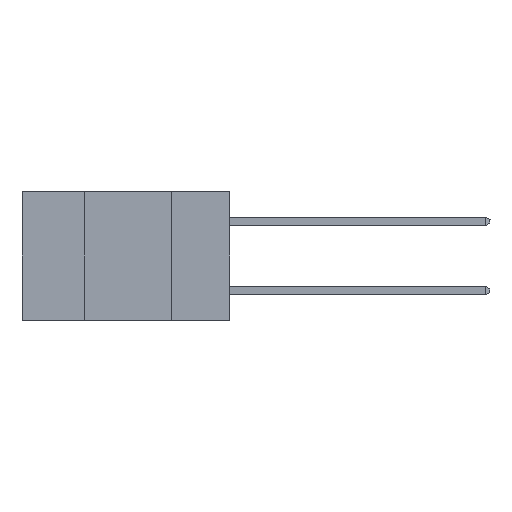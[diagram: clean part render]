
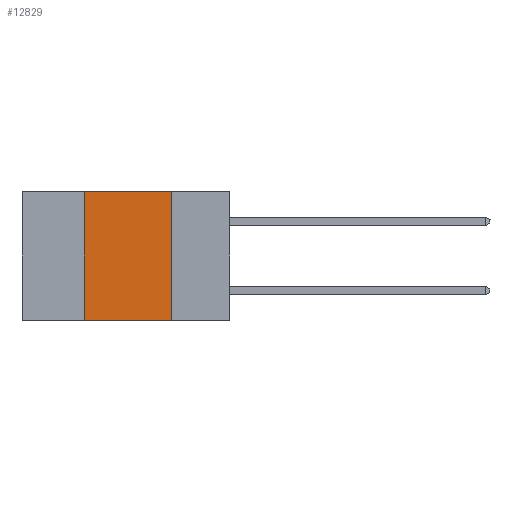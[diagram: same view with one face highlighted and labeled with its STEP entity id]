
A CAD part, left-side view. The second image highlights one B-rep face of the part: STEP entity #12829.
In plain terms, the highlighted planar face has unit normal (-1, 0, 0).
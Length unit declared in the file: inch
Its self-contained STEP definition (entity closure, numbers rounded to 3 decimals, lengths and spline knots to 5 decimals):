
#704 = DIRECTION ( 'NONE',  ( 0., 0., 1. ) ) ;
#852 = EDGE_CURVE ( 'NONE', #13391, #5458, #10496, .T. ) ;
#1098 = FACE_OUTER_BOUND ( 'NONE', #7113, .T. ) ;
#1735 = CARTESIAN_POINT ( 'NONE',  ( 0., 0.17, -0.37 ) ) ;
#2608 = ORIENTED_EDGE ( 'NONE', *, *, #852, .F. ) ;
#2869 = VERTEX_POINT ( 'NONE', #13666 ) ;
#3150 = VECTOR ( 'NONE', #5096, 39.37008 ) ;
#3332 = VERTEX_POINT ( 'NONE', #1735 ) ;
#4111 = CARTESIAN_POINT ( 'NONE',  ( 0., 0.6, 0. ) ) ;
#4150 = LINE ( 'NONE', #6909, #11896 ) ;
#4153 = DIRECTION ( 'NONE',  ( 1., 0., 0. ) ) ;
#5096 = DIRECTION ( 'NONE',  ( 0., -1., 0. ) ) ;
#5458 = VERTEX_POINT ( 'NONE', #6648 ) ;
#5935 = ORIENTED_EDGE ( 'NONE', *, *, #9139, .F. ) ;
#5999 = CARTESIAN_POINT ( 'NONE',  ( 0., 0.6, -0.37 ) ) ;
#6187 = PLANE ( 'NONE',  #8112 ) ;
#6401 = DIRECTION ( 'NONE',  ( 0., 0., -1. ) ) ;
#6648 = CARTESIAN_POINT ( 'NONE',  ( 0., 0.42, 0. ) ) ;
#6748 = VECTOR ( 'NONE', #12397, 39.37008 ) ;
#6909 = CARTESIAN_POINT ( 'NONE',  ( 0., 0.17, -0.37 ) ) ;
#7113 = EDGE_LOOP ( 'NONE', ( #10209, #5935, #2608, #13761 ) ) ;
#7265 = VECTOR ( 'NONE', #704, 39.37008 ) ;
#8112 = AXIS2_PLACEMENT_3D ( 'NONE', #13771, #4153, #6401 ) ;
#8313 = CARTESIAN_POINT ( 'NONE',  ( 0., 0.42, -0.37 ) ) ;
#8381 = CARTESIAN_POINT ( 'NONE',  ( 0., 0.42, -0.37 ) ) ;
#9139 = EDGE_CURVE ( 'NONE', #5458, #2869, #11827, .T. ) ;
#9347 = EDGE_CURVE ( 'NONE', #2869, #3332, #4150, .T. ) ;
#9441 = EDGE_CURVE ( 'NONE', #13391, #3332, #10225, .T. ) ;
#10091 = DIRECTION ( 'NONE',  ( 0., 0., -1. ) ) ;
#10209 = ORIENTED_EDGE ( 'NONE', *, *, #9347, .F. ) ;
#10225 = LINE ( 'NONE', #5999, #6748 ) ;
#10496 = LINE ( 'NONE', #8313, #7265 ) ;
#11827 = LINE ( 'NONE', #4111, #3150 ) ;
#11896 = VECTOR ( 'NONE', #10091, 39.37008 ) ;
#12397 = DIRECTION ( 'NONE',  ( 0., -1., 0. ) ) ;
#12829 = ADVANCED_FACE ( 'NONE', ( #1098 ), #6187, .F. ) ;
#13391 = VERTEX_POINT ( 'NONE', #8381 ) ;
#13666 = CARTESIAN_POINT ( 'NONE',  ( 0., 0.17, 0. ) ) ;
#13761 = ORIENTED_EDGE ( 'NONE', *, *, #9441, .T. ) ;
#13771 = CARTESIAN_POINT ( 'NONE',  ( 0., 0.6, 0. ) ) ;
